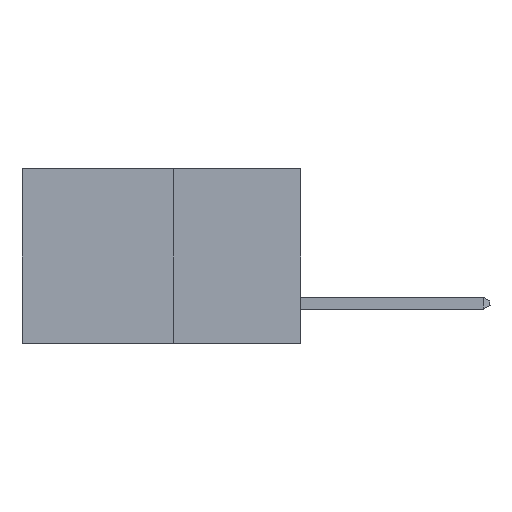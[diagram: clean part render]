
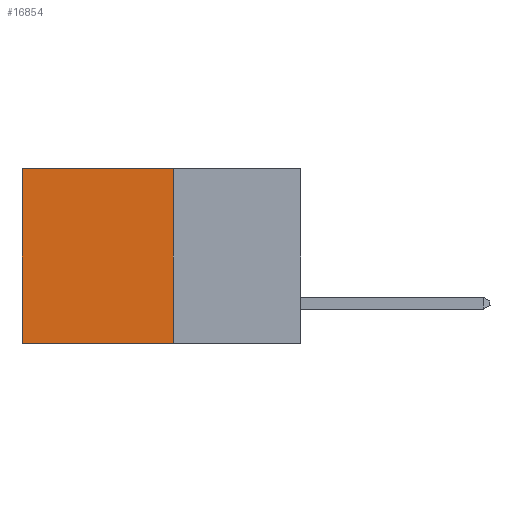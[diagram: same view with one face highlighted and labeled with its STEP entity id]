
A CAD part, left-side view. The second image highlights one B-rep face of the part: STEP entity #16854.
In plain terms, the highlighted planar face has unit normal (-1, 0, 0).
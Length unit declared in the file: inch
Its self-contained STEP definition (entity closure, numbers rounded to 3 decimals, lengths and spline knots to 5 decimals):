
#2 = EDGE_CURVE ( 'NONE', #7020, #2060, #8799, .T. ) ;
#523 = VECTOR ( 'NONE', #28843, 39.37008 ) ;
#594 = DIRECTION ( 'NONE',  ( 0., 0., -1. ) ) ;
#1066 = ORIENTED_EDGE ( 'NONE', *, *, #8456, .F. ) ;
#1656 = EDGE_LOOP ( 'NONE', ( #29173, #1066, #6183, #4440 ) ) ;
#2060 = VERTEX_POINT ( 'NONE', #16190 ) ;
#2184 = VECTOR ( 'NONE', #594, 39.37008 ) ;
#2522 = VECTOR ( 'NONE', #12235, 39.37008 ) ;
#3757 = DIRECTION ( 'NONE',  ( 0., 1., 0. ) ) ;
#4440 = ORIENTED_EDGE ( 'NONE', *, *, #11243, .T. ) ;
#4691 = PLANE ( 'NONE',  #10692 ) ;
#6183 = ORIENTED_EDGE ( 'NONE', *, *, #2, .F. ) ;
#7020 = VERTEX_POINT ( 'NONE', #15103 ) ;
#7241 = CARTESIAN_POINT ( 'NONE',  ( 0.277, 0.59, -0.37 ) ) ;
#7533 = LINE ( 'NONE', #7564, #523 ) ;
#7564 = CARTESIAN_POINT ( 'NONE',  ( 0.277, 0.27, 0. ) ) ;
#8372 = FACE_OUTER_BOUND ( 'NONE', #1656, .T. ) ;
#8456 = EDGE_CURVE ( 'NONE', #2060, #17535, #22132, .T. ) ;
#8799 = LINE ( 'NONE', #25469, #2522 ) ;
#9435 = CARTESIAN_POINT ( 'NONE',  ( 0.277, 0.27, -0.37 ) ) ;
#9541 = VECTOR ( 'NONE', #3757, 39.37008 ) ;
#10692 = AXIS2_PLACEMENT_3D ( 'NONE', #9435, #25974, #11809 ) ;
#11243 = EDGE_CURVE ( 'NONE', #7020, #23912, #7533, .T. ) ;
#11809 = DIRECTION ( 'NONE',  ( 0., 0., -1. ) ) ;
#12235 = DIRECTION ( 'NONE',  ( 0., 0., -1. ) ) ;
#14751 = CARTESIAN_POINT ( 'NONE',  ( 0.277, 0.59, -0.37 ) ) ;
#15103 = CARTESIAN_POINT ( 'NONE',  ( 0.277, 0.27, 0. ) ) ;
#16190 = CARTESIAN_POINT ( 'NONE',  ( 0.277, 0.27, -0.37 ) ) ;
#16854 = ADVANCED_FACE ( 'NONE', ( #8372 ), #4691, .F. ) ;
#17535 = VERTEX_POINT ( 'NONE', #7241 ) ;
#21844 = EDGE_CURVE ( 'NONE', #23912, #17535, #26556, .T. ) ;
#22132 = LINE ( 'NONE', #22672, #9541 ) ;
#22672 = CARTESIAN_POINT ( 'NONE',  ( 0.277, 0.27, -0.37 ) ) ;
#23912 = VERTEX_POINT ( 'NONE', #24749 ) ;
#24749 = CARTESIAN_POINT ( 'NONE',  ( 0.277, 0.59, 0. ) ) ;
#25469 = CARTESIAN_POINT ( 'NONE',  ( 0.277, 0.27, -0.37 ) ) ;
#25974 = DIRECTION ( 'NONE',  ( 1., 0., 0. ) ) ;
#26556 = LINE ( 'NONE', #14751, #2184 ) ;
#28843 = DIRECTION ( 'NONE',  ( 0., 1., 0. ) ) ;
#29173 = ORIENTED_EDGE ( 'NONE', *, *, #21844, .T. ) ;
